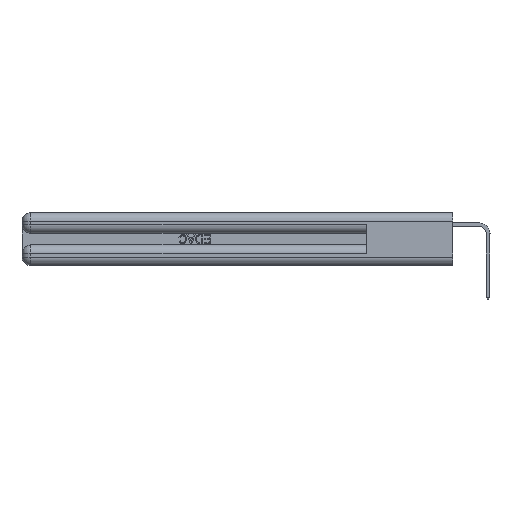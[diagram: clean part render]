
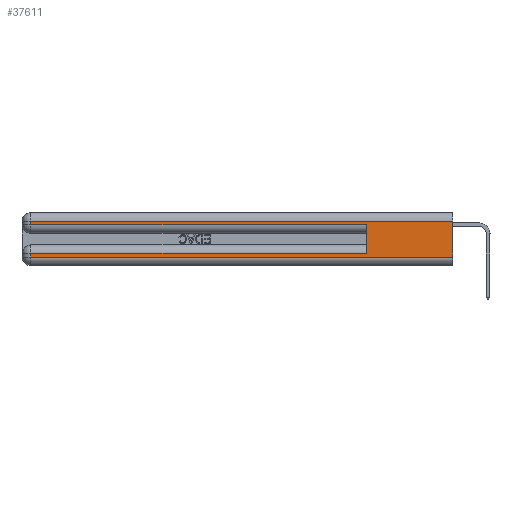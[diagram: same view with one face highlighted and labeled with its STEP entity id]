
A CAD part, left-side view. The second image highlights one B-rep face of the part: STEP entity #37611.
In plain terms, the highlighted planar face has unit normal (-1, 0, 0).
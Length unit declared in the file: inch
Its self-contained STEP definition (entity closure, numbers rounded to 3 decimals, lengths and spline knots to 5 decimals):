
#946 = VECTOR ( 'NONE', #20409, 39.37008 ) ;
#2743 = VECTOR ( 'NONE', #35750, 39.37008 ) ;
#4002 = DIRECTION ( 'NONE',  ( 1., 0., 0. ) ) ;
#4445 = CARTESIAN_POINT ( 'NONE',  ( 0., 2.94, 0.285 ) ) ;
#5388 = EDGE_CURVE ( 'NONE', #40875, #16911, #9612, .T. ) ;
#6180 = EDGE_CURVE ( 'NONE', #18877, #16911, #21178, .T. ) ;
#6351 = ORIENTED_EDGE ( 'NONE', *, *, #6180, .F. ) ;
#6446 = ORIENTED_EDGE ( 'NONE', *, *, #5388, .T. ) ;
#6658 = LINE ( 'NONE', #14075, #31300 ) ;
#7038 = DIRECTION ( 'NONE',  ( 0., 0., -1. ) ) ;
#7604 = ORIENTED_EDGE ( 'NONE', *, *, #40432, .T. ) ;
#8236 = VECTOR ( 'NONE', #25438, 39.37008 ) ;
#8446 = LINE ( 'NONE', #39390, #946 ) ;
#9386 = CARTESIAN_POINT ( 'NONE',  ( 0., 0.6, 0.145 ) ) ;
#9612 = LINE ( 'NONE', #17470, #17233 ) ;
#9779 = DIRECTION ( 'NONE',  ( 0., -1., 0. ) ) ;
#10794 = DIRECTION ( 'NONE',  ( 0., -1., 0. ) ) ;
#11294 = LINE ( 'NONE', #19802, #2743 ) ;
#12748 = CARTESIAN_POINT ( 'NONE',  ( 0., 0., 0.31 ) ) ;
#14075 = CARTESIAN_POINT ( 'NONE',  ( 0., 0., 0.085 ) ) ;
#14820 = EDGE_CURVE ( 'NONE', #18877, #23655, #8446, .T. ) ;
#15367 = ORIENTED_EDGE ( 'NONE', *, *, #14820, .T. ) ;
#15392 = CARTESIAN_POINT ( 'NONE',  ( 0., 0., 0.37 ) ) ;
#15827 = CARTESIAN_POINT ( 'NONE',  ( 0., 2.94, 0.085 ) ) ;
#15833 = FACE_OUTER_BOUND ( 'NONE', #21990, .T. ) ;
#16510 = CARTESIAN_POINT ( 'NONE',  ( 0., 2.94, 0.06 ) ) ;
#16843 = PLANE ( 'NONE',  #30869 ) ;
#16911 = VERTEX_POINT ( 'NONE', #38387 ) ;
#17037 = EDGE_CURVE ( 'NONE', #23655, #19130, #11294, .T. ) ;
#17233 = VECTOR ( 'NONE', #10794, 39.37008 ) ;
#17358 = DIRECTION ( 'NONE',  ( 0., 1., 0. ) ) ;
#17470 = CARTESIAN_POINT ( 'NONE',  ( 0., 0., 0.06 ) ) ;
#18877 = VERTEX_POINT ( 'NONE', #12748 ) ;
#19130 = VERTEX_POINT ( 'NONE', #4445 ) ;
#19236 = LINE ( 'NONE', #38919, #25716 ) ;
#19523 = VERTEX_POINT ( 'NONE', #15827 ) ;
#19802 = CARTESIAN_POINT ( 'NONE',  ( 0., 2.94, 0.37 ) ) ;
#20409 = DIRECTION ( 'NONE',  ( 0., 1., 0. ) ) ;
#21178 = LINE ( 'NONE', #15392, #37047 ) ;
#21990 = EDGE_LOOP ( 'NONE', ( #6351, #15367, #39768, #38674, #28781, #27945, #7604, #6446 ) ) ;
#22103 = LINE ( 'NONE', #25838, #23117 ) ;
#23117 = VECTOR ( 'NONE', #9779, 39.37008 ) ;
#23309 = CARTESIAN_POINT ( 'NONE',  ( 0., 0., 0.37 ) ) ;
#23655 = VERTEX_POINT ( 'NONE', #25225 ) ;
#25225 = CARTESIAN_POINT ( 'NONE',  ( 0., 2.94, 0.31 ) ) ;
#25438 = DIRECTION ( 'NONE',  ( 0., 0., 1. ) ) ;
#25716 = VECTOR ( 'NONE', #7038, 39.37008 ) ;
#25838 = CARTESIAN_POINT ( 'NONE',  ( 0., 0., 0.285 ) ) ;
#26524 = DIRECTION ( 'NONE',  ( 0., 0., -1. ) ) ;
#27741 = EDGE_CURVE ( 'NONE', #19130, #30511, #22103, .T. ) ;
#27945 = ORIENTED_EDGE ( 'NONE', *, *, #38340, .T. ) ;
#28781 = ORIENTED_EDGE ( 'NONE', *, *, #34096, .F. ) ;
#30511 = VERTEX_POINT ( 'NONE', #32208 ) ;
#30869 = AXIS2_PLACEMENT_3D ( 'NONE', #23309, #4002, #26524 ) ;
#31300 = VECTOR ( 'NONE', #17358, 39.37008 ) ;
#32208 = CARTESIAN_POINT ( 'NONE',  ( 0., 0.6, 0.285 ) ) ;
#32399 = VERTEX_POINT ( 'NONE', #38822 ) ;
#34096 = EDGE_CURVE ( 'NONE', #32399, #30511, #41214, .T. ) ;
#35750 = DIRECTION ( 'NONE',  ( 0., 0., -1. ) ) ;
#37047 = VECTOR ( 'NONE', #40848, 39.37008 ) ;
#37611 = ADVANCED_FACE ( 'NONE', ( #15833 ), #16843, .F. ) ;
#38340 = EDGE_CURVE ( 'NONE', #32399, #19523, #6658, .T. ) ;
#38387 = CARTESIAN_POINT ( 'NONE',  ( 0., 0., 0.06 ) ) ;
#38674 = ORIENTED_EDGE ( 'NONE', *, *, #27741, .T. ) ;
#38822 = CARTESIAN_POINT ( 'NONE',  ( 0., 0.6, 0.085 ) ) ;
#38919 = CARTESIAN_POINT ( 'NONE',  ( 0., 2.94, 0.37 ) ) ;
#39390 = CARTESIAN_POINT ( 'NONE',  ( 0., 0., 0.31 ) ) ;
#39768 = ORIENTED_EDGE ( 'NONE', *, *, #17037, .T. ) ;
#40432 = EDGE_CURVE ( 'NONE', #19523, #40875, #19236, .T. ) ;
#40848 = DIRECTION ( 'NONE',  ( 0., 0., -1. ) ) ;
#40875 = VERTEX_POINT ( 'NONE', #16510 ) ;
#41214 = LINE ( 'NONE', #9386, #8236 ) ;
